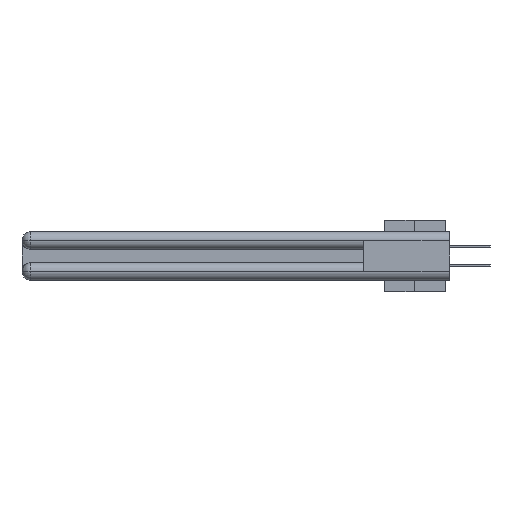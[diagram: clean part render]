
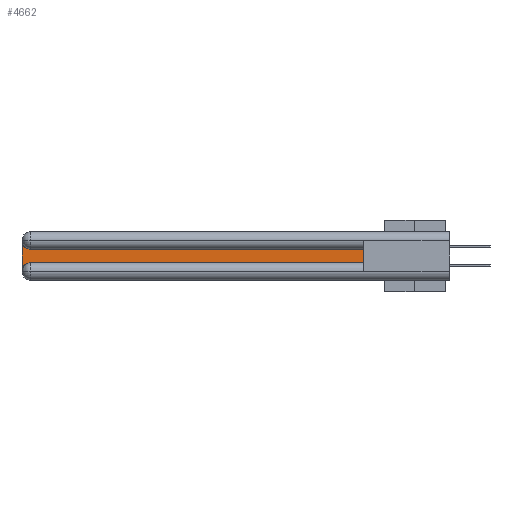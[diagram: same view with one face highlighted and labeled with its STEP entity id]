
A CAD part, left-side view. The second image highlights one B-rep face of the part: STEP entity #4662.
In plain terms, the highlighted planar face has unit normal (-1, 0, 0).
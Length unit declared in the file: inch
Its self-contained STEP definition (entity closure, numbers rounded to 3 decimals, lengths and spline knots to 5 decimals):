
#142 = ORIENTED_EDGE ( 'NONE', *, *, #28695, .T. ) ;
#309 = DIRECTION ( 'NONE',  ( 1., 0., 0. ) ) ;
#952 = AXIS2_PLACEMENT_3D ( 'NONE', #23201, #9476, #31479 ) ;
#1860 = EDGE_CURVE ( 'NONE', #27179, #26530, #19283, .T. ) ;
#2620 = CARTESIAN_POINT ( 'NONE',  ( 0.075, 2.94, -0.1225 ) ) ;
#3558 = CARTESIAN_POINT ( 'NONE',  ( 0.075, 0.6, -0.1225 ) ) ;
#3742 = DIRECTION ( 'NONE',  ( 0., -1., 0. ) ) ;
#4662 = ADVANCED_FACE ( 'NONE', ( #18565 ), #17632, .F. ) ;
#4956 = AXIS2_PLACEMENT_3D ( 'NONE', #23787, #29066, #16283 ) ;
#5149 = VECTOR ( 'NONE', #8824, 39.37008 ) ;
#8066 = ORIENTED_EDGE ( 'NONE', *, *, #31287, .T. ) ;
#8286 = EDGE_CURVE ( 'NONE', #21171, #35233, #15221, .T. ) ;
#8824 = DIRECTION ( 'NONE',  ( 0., 1., 0. ) ) ;
#8971 = VECTOR ( 'NONE', #34962, 39.37008 ) ;
#9476 = DIRECTION ( 'NONE',  ( 1., 0., 0. ) ) ;
#9895 = CARTESIAN_POINT ( 'NONE',  ( 0.075, 2.94, -0.2175 ) ) ;
#10220 = ORIENTED_EDGE ( 'NONE', *, *, #1860, .T. ) ;
#10269 = LINE ( 'NONE', #25722, #31376 ) ;
#11558 = VECTOR ( 'NONE', #13343, 39.37008 ) ;
#11969 = ORIENTED_EDGE ( 'NONE', *, *, #19653, .T. ) ;
#12418 = LINE ( 'NONE', #29613, #11558 ) ;
#13343 = DIRECTION ( 'NONE',  ( 0., 0., 1. ) ) ;
#14121 = VERTEX_POINT ( 'NONE', #20596 ) ;
#15221 = CIRCLE ( 'NONE', #4956, 0.06 ) ;
#15410 = LINE ( 'NONE', #21269, #8971 ) ;
#16283 = DIRECTION ( 'NONE',  ( 0., 0., -1. ) ) ;
#17632 = PLANE ( 'NONE',  #952 ) ;
#18565 = FACE_OUTER_BOUND ( 'NONE', #27531, .T. ) ;
#18916 = ORIENTED_EDGE ( 'NONE', *, *, #28297, .T. ) ;
#19283 = CIRCLE ( 'NONE', #28771, 0.06 ) ;
#19286 = CARTESIAN_POINT ( 'NONE',  ( 0.075, 3., -0.0625 ) ) ;
#19653 = EDGE_CURVE ( 'NONE', #26530, #14121, #10269, .T. ) ;
#20572 = CARTESIAN_POINT ( 'NONE',  ( 0.075, 3., -0.2775 ) ) ;
#20596 = CARTESIAN_POINT ( 'NONE',  ( 0.075, 0.6, -0.2175 ) ) ;
#21171 = VERTEX_POINT ( 'NONE', #2620 ) ;
#21269 = CARTESIAN_POINT ( 'NONE',  ( 0.075, 3., -0.2175 ) ) ;
#22333 = DIRECTION ( 'NONE',  ( 0., 0., -1. ) ) ;
#23056 = CARTESIAN_POINT ( 'NONE',  ( 0.075, 2.94, -0.2775 ) ) ;
#23201 = CARTESIAN_POINT ( 'NONE',  ( 0.075, 3., -0.1225 ) ) ;
#23787 = CARTESIAN_POINT ( 'NONE',  ( 0.075, 2.94, -0.0625 ) ) ;
#25349 = VERTEX_POINT ( 'NONE', #29796 ) ;
#25722 = CARTESIAN_POINT ( 'NONE',  ( 0.075, 0.6, -0.2175 ) ) ;
#26250 = LINE ( 'NONE', #3558, #5149 ) ;
#26530 = VERTEX_POINT ( 'NONE', #9895 ) ;
#27179 = VERTEX_POINT ( 'NONE', #20572 ) ;
#27531 = EDGE_LOOP ( 'NONE', ( #18916, #33645, #8066, #10220, #11969, #142 ) ) ;
#28297 = EDGE_CURVE ( 'NONE', #25349, #21171, #26250, .T. ) ;
#28695 = EDGE_CURVE ( 'NONE', #14121, #25349, #12418, .T. ) ;
#28771 = AXIS2_PLACEMENT_3D ( 'NONE', #23056, #309, #22333 ) ;
#29066 = DIRECTION ( 'NONE',  ( 1., 0., 0. ) ) ;
#29613 = CARTESIAN_POINT ( 'NONE',  ( 0.075, 0.6, -0.2175 ) ) ;
#29796 = CARTESIAN_POINT ( 'NONE',  ( 0.075, 0.6, -0.1225 ) ) ;
#31287 = EDGE_CURVE ( 'NONE', #35233, #27179, #15410, .T. ) ;
#31376 = VECTOR ( 'NONE', #3742, 39.37008 ) ;
#31479 = DIRECTION ( 'NONE',  ( 0., 0., -1. ) ) ;
#33645 = ORIENTED_EDGE ( 'NONE', *, *, #8286, .T. ) ;
#34962 = DIRECTION ( 'NONE',  ( 0., 0., -1. ) ) ;
#35233 = VERTEX_POINT ( 'NONE', #19286 ) ;
